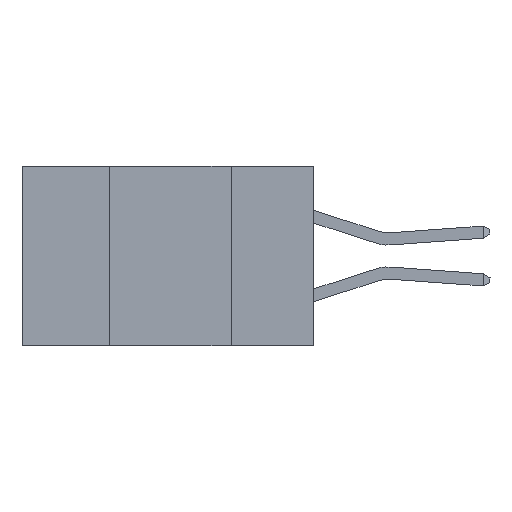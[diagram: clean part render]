
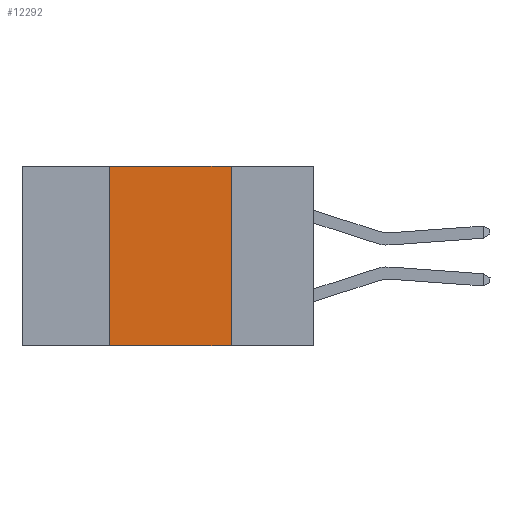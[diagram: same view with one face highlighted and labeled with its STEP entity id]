
A CAD part, left-side view. The second image highlights one B-rep face of the part: STEP entity #12292.
In plain terms, the highlighted planar face has unit normal (-1, 0, 0).
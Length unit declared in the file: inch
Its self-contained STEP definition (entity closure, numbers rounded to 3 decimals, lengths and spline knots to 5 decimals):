
#772 = ORIENTED_EDGE ( 'NONE', *, *, #12450, .F. ) ;
#1475 = LINE ( 'NONE', #8555, #9006 ) ;
#2311 = DIRECTION ( 'NONE',  ( 1., 0., 0. ) ) ;
#2458 = DIRECTION ( 'NONE',  ( 0., 0., 1. ) ) ;
#2563 = CARTESIAN_POINT ( 'NONE',  ( 0., 0.17, 0. ) ) ;
#3113 = VERTEX_POINT ( 'NONE', #6632 ) ;
#3163 = CARTESIAN_POINT ( 'NONE',  ( 0., 0.42, -0.37 ) ) ;
#3265 = CARTESIAN_POINT ( 'NONE',  ( 0., 0.6, -0.37 ) ) ;
#3701 = EDGE_CURVE ( 'NONE', #4385, #7516, #1475, .T. ) ;
#3871 = VECTOR ( 'NONE', #12725, 39.37008 ) ;
#4385 = VERTEX_POINT ( 'NONE', #2563 ) ;
#4655 = FACE_OUTER_BOUND ( 'NONE', #7701, .T. ) ;
#6443 = PLANE ( 'NONE',  #8888 ) ;
#6632 = CARTESIAN_POINT ( 'NONE',  ( 0., 0.42, 0. ) ) ;
#7201 = LINE ( 'NONE', #3265, #11650 ) ;
#7516 = VERTEX_POINT ( 'NONE', #12727 ) ;
#7701 = EDGE_LOOP ( 'NONE', ( #8004, #8303, #772, #8455 ) ) ;
#7869 = DIRECTION ( 'NONE',  ( 0., 0., -1. ) ) ;
#8004 = ORIENTED_EDGE ( 'NONE', *, *, #3701, .F. ) ;
#8294 = EDGE_CURVE ( 'NONE', #10717, #7516, #7201, .T. ) ;
#8303 = ORIENTED_EDGE ( 'NONE', *, *, #11340, .F. ) ;
#8448 = CARTESIAN_POINT ( 'NONE',  ( 0., 0.6, 0. ) ) ;
#8455 = ORIENTED_EDGE ( 'NONE', *, *, #8294, .T. ) ;
#8555 = CARTESIAN_POINT ( 'NONE',  ( 0., 0.17, 0. ) ) ;
#8614 = CARTESIAN_POINT ( 'NONE',  ( 0., 0.42, 0. ) ) ;
#8888 = AXIS2_PLACEMENT_3D ( 'NONE', #8448, #2311, #9408 ) ;
#8909 = VECTOR ( 'NONE', #2458, 39.37008 ) ;
#9006 = VECTOR ( 'NONE', #7869, 39.37008 ) ;
#9203 = LINE ( 'NONE', #10868, #3871 ) ;
#9408 = DIRECTION ( 'NONE',  ( 0., 0., -1. ) ) ;
#10717 = VERTEX_POINT ( 'NONE', #3163 ) ;
#10868 = CARTESIAN_POINT ( 'NONE',  ( 0., 0.6, 0. ) ) ;
#11340 = EDGE_CURVE ( 'NONE', #3113, #4385, #9203, .T. ) ;
#11650 = VECTOR ( 'NONE', #12085, 39.37008 ) ;
#11663 = LINE ( 'NONE', #8614, #8909 ) ;
#12085 = DIRECTION ( 'NONE',  ( 0., -1., 0. ) ) ;
#12292 = ADVANCED_FACE ( 'NONE', ( #4655 ), #6443, .F. ) ;
#12450 = EDGE_CURVE ( 'NONE', #10717, #3113, #11663, .T. ) ;
#12725 = DIRECTION ( 'NONE',  ( 0., -1., 0. ) ) ;
#12727 = CARTESIAN_POINT ( 'NONE',  ( 0., 0.17, -0.37 ) ) ;
